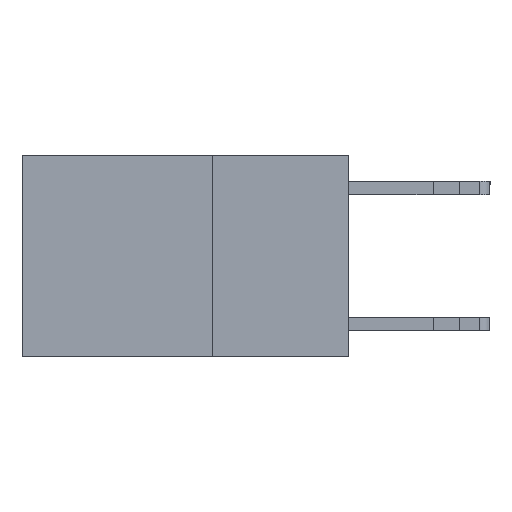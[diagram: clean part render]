
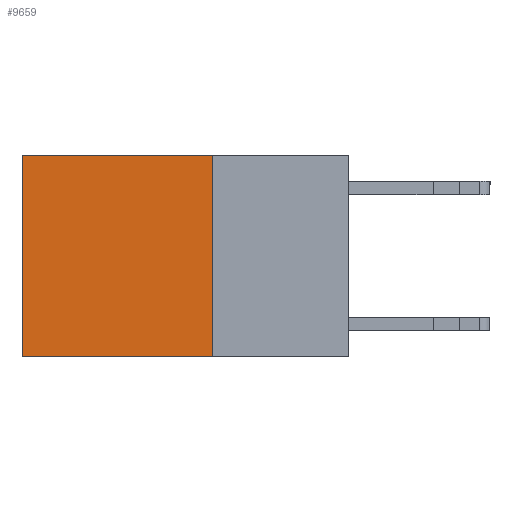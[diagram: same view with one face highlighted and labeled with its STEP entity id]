
A CAD part, left-side view. The second image highlights one B-rep face of the part: STEP entity #9659.
In plain terms, the highlighted planar face has unit normal (-1, 0, 0).
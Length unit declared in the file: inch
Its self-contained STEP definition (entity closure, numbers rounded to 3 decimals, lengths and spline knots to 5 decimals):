
#3 = DIRECTION ( 'NONE',  ( 1., 0., 0. ) ) ;
#15 = VECTOR ( 'NONE', #9419, 39.37008 ) ;
#93 = CARTESIAN_POINT ( 'NONE',  ( 0.2625, 0.25, -0.37 ) ) ;
#601 = EDGE_CURVE ( 'NONE', #1300, #4908, #3351, .T. ) ;
#684 = CARTESIAN_POINT ( 'NONE',  ( 0.2625, 0.6, 0. ) ) ;
#811 = LINE ( 'NONE', #2064, #6937 ) ;
#864 = EDGE_LOOP ( 'NONE', ( #11927, #5768, #4625, #3244 ) ) ;
#1300 = VERTEX_POINT ( 'NONE', #684 ) ;
#2064 = CARTESIAN_POINT ( 'NONE',  ( 0.2625, 0.25, 0. ) ) ;
#2260 = DIRECTION ( 'NONE',  ( 0., 0., -1. ) ) ;
#2293 = LINE ( 'NONE', #8034, #12386 ) ;
#2629 = VECTOR ( 'NONE', #2260, 39.37008 ) ;
#2900 = EDGE_CURVE ( 'NONE', #9573, #13381, #9651, .T. ) ;
#3229 = CARTESIAN_POINT ( 'NONE',  ( 0.2625, 0.25, 0. ) ) ;
#3244 = ORIENTED_EDGE ( 'NONE', *, *, #14246, .T. ) ;
#3351 = LINE ( 'NONE', #4520, #2629 ) ;
#3673 = DIRECTION ( 'NONE',  ( 0., 1., 0. ) ) ;
#3968 = EDGE_CURVE ( 'NONE', #13381, #4908, #2293, .T. ) ;
#4459 = DIRECTION ( 'NONE',  ( 0., 0., -1. ) ) ;
#4520 = CARTESIAN_POINT ( 'NONE',  ( 0.2625, 0.6, 0. ) ) ;
#4625 = ORIENTED_EDGE ( 'NONE', *, *, #2900, .F. ) ;
#4908 = VERTEX_POINT ( 'NONE', #6984 ) ;
#5486 = AXIS2_PLACEMENT_3D ( 'NONE', #3229, #3, #4459 ) ;
#5768 = ORIENTED_EDGE ( 'NONE', *, *, #3968, .F. ) ;
#6004 = CARTESIAN_POINT ( 'NONE',  ( 0.2625, 0.25, 0. ) ) ;
#6576 = DIRECTION ( 'NONE',  ( 0., 1., 0. ) ) ;
#6937 = VECTOR ( 'NONE', #6576, 39.37008 ) ;
#6984 = CARTESIAN_POINT ( 'NONE',  ( 0.2625, 0.6, -0.37 ) ) ;
#8034 = CARTESIAN_POINT ( 'NONE',  ( 0.2625, 0.25, -0.37 ) ) ;
#8896 = FACE_OUTER_BOUND ( 'NONE', #864, .T. ) ;
#9419 = DIRECTION ( 'NONE',  ( 0., 0., -1. ) ) ;
#9573 = VERTEX_POINT ( 'NONE', #12844 ) ;
#9651 = LINE ( 'NONE', #6004, #15 ) ;
#9659 = ADVANCED_FACE ( 'NONE', ( #8896 ), #9998, .F. ) ;
#9998 = PLANE ( 'NONE',  #5486 ) ;
#11927 = ORIENTED_EDGE ( 'NONE', *, *, #601, .T. ) ;
#12386 = VECTOR ( 'NONE', #3673, 39.37008 ) ;
#12844 = CARTESIAN_POINT ( 'NONE',  ( 0.2625, 0.25, 0. ) ) ;
#13381 = VERTEX_POINT ( 'NONE', #93 ) ;
#14246 = EDGE_CURVE ( 'NONE', #9573, #1300, #811, .T. ) ;
